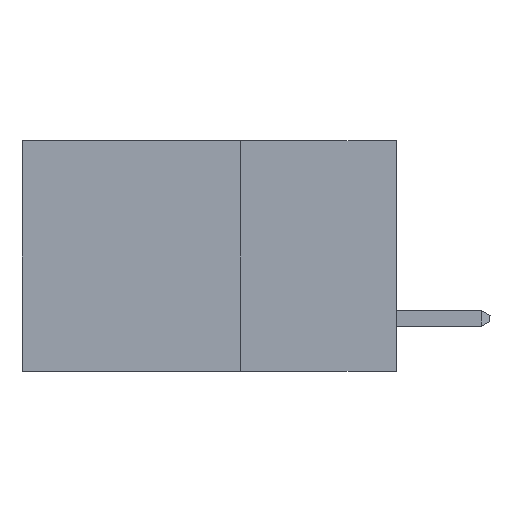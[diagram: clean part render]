
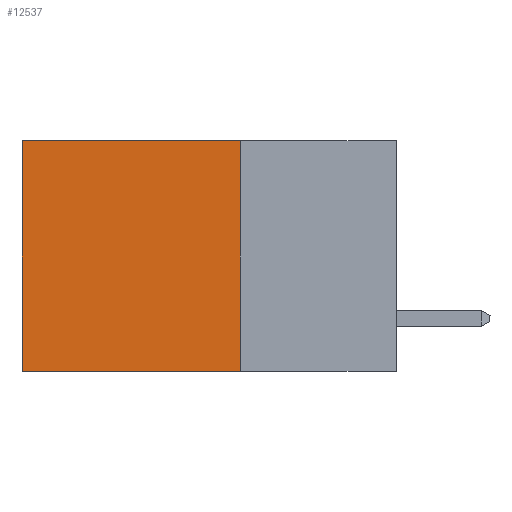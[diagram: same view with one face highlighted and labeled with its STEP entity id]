
A CAD part, left-side view. The second image highlights one B-rep face of the part: STEP entity #12537.
In plain terms, the highlighted planar face has unit normal (-1, 0, 0).
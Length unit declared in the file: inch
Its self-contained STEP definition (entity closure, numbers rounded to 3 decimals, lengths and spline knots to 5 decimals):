
#713 = CARTESIAN_POINT ( 'NONE',  ( 0.2615, 0.25, -0.37 ) ) ;
#1583 = EDGE_CURVE ( 'NONE', #10290, #19612, #11345, .T. ) ;
#3567 = ORIENTED_EDGE ( 'NONE', *, *, #12456, .T. ) ;
#4586 = CARTESIAN_POINT ( 'NONE',  ( 0.2615, 0.6, 0. ) ) ;
#5058 = DIRECTION ( 'NONE',  ( 0., 0., -1. ) ) ;
#5259 = CARTESIAN_POINT ( 'NONE',  ( 0.2615, 0.25, -0.37 ) ) ;
#5290 = EDGE_CURVE ( 'NONE', #10290, #16927, #16065, .T. ) ;
#6723 = VECTOR ( 'NONE', #13031, 39.37008 ) ;
#7177 = CARTESIAN_POINT ( 'NONE',  ( 0.2615, 0.6, -0.37 ) ) ;
#7214 = LINE ( 'NONE', #20215, #11746 ) ;
#10042 = DIRECTION ( 'NONE',  ( 0., 0., -1. ) ) ;
#10290 = VERTEX_POINT ( 'NONE', #15907 ) ;
#11242 = LINE ( 'NONE', #18090, #6723 ) ;
#11345 = LINE ( 'NONE', #5259, #19851 ) ;
#11439 = DIRECTION ( 'NONE',  ( 1., 0., 0. ) ) ;
#11746 = VECTOR ( 'NONE', #10042, 39.37008 ) ;
#11796 = EDGE_CURVE ( 'NONE', #19612, #14529, #11242, .T. ) ;
#11985 = DIRECTION ( 'NONE',  ( 0., 0., -1. ) ) ;
#12126 = AXIS2_PLACEMENT_3D ( 'NONE', #18729, #11439, #11985 ) ;
#12387 = EDGE_LOOP ( 'NONE', ( #3567, #14416, #13642, #14369 ) ) ;
#12456 = EDGE_CURVE ( 'NONE', #16927, #14529, #7214, .T. ) ;
#12537 = ADVANCED_FACE ( 'NONE', ( #15230 ), #15344, .F. ) ;
#13031 = DIRECTION ( 'NONE',  ( 0., 1., 0. ) ) ;
#13642 = ORIENTED_EDGE ( 'NONE', *, *, #1583, .F. ) ;
#14369 = ORIENTED_EDGE ( 'NONE', *, *, #5290, .T. ) ;
#14416 = ORIENTED_EDGE ( 'NONE', *, *, #11796, .F. ) ;
#14529 = VERTEX_POINT ( 'NONE', #7177 ) ;
#14977 = VECTOR ( 'NONE', #21624, 39.37008 ) ;
#15230 = FACE_OUTER_BOUND ( 'NONE', #12387, .T. ) ;
#15344 = PLANE ( 'NONE',  #12126 ) ;
#15907 = CARTESIAN_POINT ( 'NONE',  ( 0.2615, 0.25, 0. ) ) ;
#16065 = LINE ( 'NONE', #21617, #14977 ) ;
#16927 = VERTEX_POINT ( 'NONE', #4586 ) ;
#18090 = CARTESIAN_POINT ( 'NONE',  ( 0.2615, 0.25, -0.37 ) ) ;
#18729 = CARTESIAN_POINT ( 'NONE',  ( 0.2615, 0.25, -0.37 ) ) ;
#19612 = VERTEX_POINT ( 'NONE', #713 ) ;
#19851 = VECTOR ( 'NONE', #5058, 39.37008 ) ;
#20215 = CARTESIAN_POINT ( 'NONE',  ( 0.2615, 0.6, -0.37 ) ) ;
#21617 = CARTESIAN_POINT ( 'NONE',  ( 0.2615, 0.25, 0. ) ) ;
#21624 = DIRECTION ( 'NONE',  ( 0., 1., 0. ) ) ;
